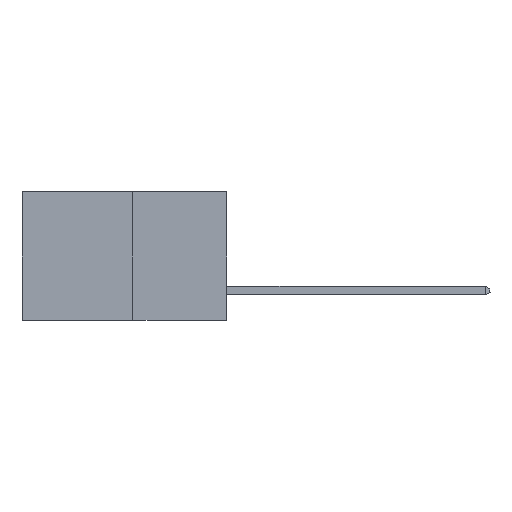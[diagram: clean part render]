
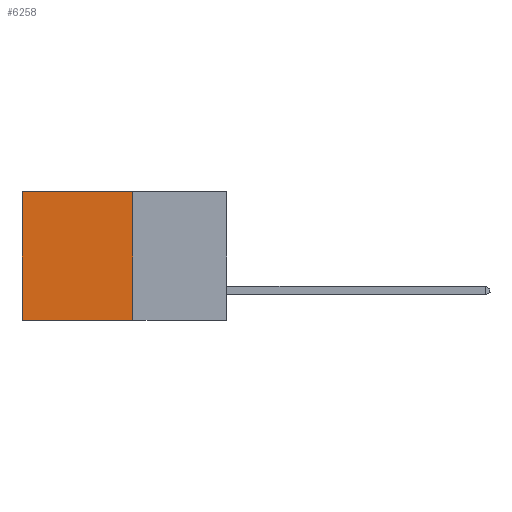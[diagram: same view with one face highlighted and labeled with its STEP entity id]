
A CAD part, left-side view. The second image highlights one B-rep face of the part: STEP entity #6258.
In plain terms, the highlighted planar face has unit normal (-1, 0, 0).
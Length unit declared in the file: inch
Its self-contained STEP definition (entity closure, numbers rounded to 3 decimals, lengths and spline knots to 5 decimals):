
#102 = VERTEX_POINT ( 'NONE', #138 ) ;
#138 = CARTESIAN_POINT ( 'NONE',  ( 0.277, 0.27, -0.37 ) ) ;
#473 = VECTOR ( 'NONE', #4221, 39.37008 ) ;
#1444 = VECTOR ( 'NONE', #11725, 39.37008 ) ;
#1685 = VERTEX_POINT ( 'NONE', #5484 ) ;
#2686 = CARTESIAN_POINT ( 'NONE',  ( 0.277, 0.27, -0.37 ) ) ;
#2974 = CARTESIAN_POINT ( 'NONE',  ( 0.277, 0.59, -0.37 ) ) ;
#3017 = CARTESIAN_POINT ( 'NONE',  ( 0.277, 0.27, -0.37 ) ) ;
#3730 = FACE_OUTER_BOUND ( 'NONE', #9963, .T. ) ;
#3885 = DIRECTION ( 'NONE',  ( 0., 0., -1. ) ) ;
#4124 = EDGE_CURVE ( 'NONE', #12361, #102, #6527, .T. ) ;
#4149 = DIRECTION ( 'NONE',  ( 0., 1., 0. ) ) ;
#4221 = DIRECTION ( 'NONE',  ( 0., 0., -1. ) ) ;
#4593 = EDGE_CURVE ( 'NONE', #102, #10405, #6851, .T. ) ;
#4758 = CARTESIAN_POINT ( 'NONE',  ( 0.277, 0.27, 0. ) ) ;
#5179 = CARTESIAN_POINT ( 'NONE',  ( 0.277, 0.27, -0.37 ) ) ;
#5311 = EDGE_CURVE ( 'NONE', #12361, #1685, #7300, .T. ) ;
#5484 = CARTESIAN_POINT ( 'NONE',  ( 0.277, 0.59, 0. ) ) ;
#5978 = ORIENTED_EDGE ( 'NONE', *, *, #9762, .T. ) ;
#6258 = ADVANCED_FACE ( 'NONE', ( #3730 ), #7942, .F. ) ;
#6527 = LINE ( 'NONE', #3017, #473 ) ;
#6851 = LINE ( 'NONE', #5179, #11870 ) ;
#7300 = LINE ( 'NONE', #4758, #1444 ) ;
#7461 = ORIENTED_EDGE ( 'NONE', *, *, #5311, .T. ) ;
#7885 = CARTESIAN_POINT ( 'NONE',  ( 0.277, 0.27, 0. ) ) ;
#7907 = CARTESIAN_POINT ( 'NONE',  ( 0.277, 0.59, -0.37 ) ) ;
#7942 = PLANE ( 'NONE',  #10433 ) ;
#7989 = ORIENTED_EDGE ( 'NONE', *, *, #4124, .F. ) ;
#8652 = VECTOR ( 'NONE', #12187, 39.37008 ) ;
#9754 = ORIENTED_EDGE ( 'NONE', *, *, #4593, .F. ) ;
#9762 = EDGE_CURVE ( 'NONE', #1685, #10405, #10759, .T. ) ;
#9936 = DIRECTION ( 'NONE',  ( 1., 0., 0. ) ) ;
#9963 = EDGE_LOOP ( 'NONE', ( #5978, #9754, #7989, #7461 ) ) ;
#10405 = VERTEX_POINT ( 'NONE', #7907 ) ;
#10433 = AXIS2_PLACEMENT_3D ( 'NONE', #2686, #9936, #3885 ) ;
#10759 = LINE ( 'NONE', #2974, #8652 ) ;
#11725 = DIRECTION ( 'NONE',  ( 0., 1., 0. ) ) ;
#11870 = VECTOR ( 'NONE', #4149, 39.37008 ) ;
#12187 = DIRECTION ( 'NONE',  ( 0., 0., -1. ) ) ;
#12361 = VERTEX_POINT ( 'NONE', #7885 ) ;
